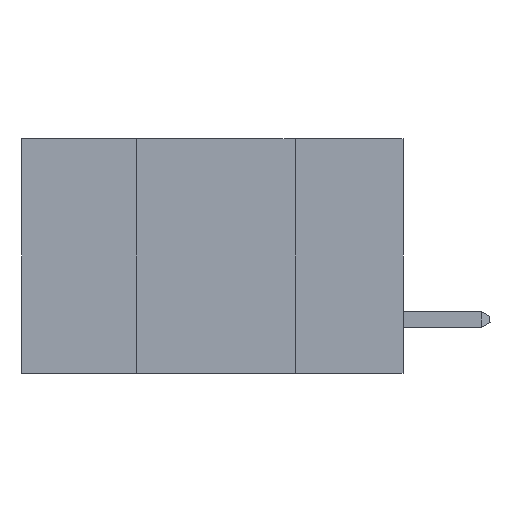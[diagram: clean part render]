
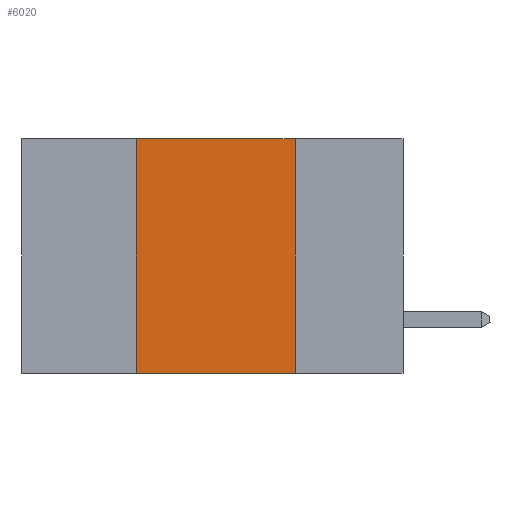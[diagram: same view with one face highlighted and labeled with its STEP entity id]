
A CAD part, left-side view. The second image highlights one B-rep face of the part: STEP entity #6020.
In plain terms, the highlighted planar face has unit normal (-1, 0, 0).
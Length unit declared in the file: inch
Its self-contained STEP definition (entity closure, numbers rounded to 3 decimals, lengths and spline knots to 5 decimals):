
#1434 = LINE ( 'NONE', #20074, #16120 ) ;
#2878 = EDGE_CURVE ( 'NONE', #14919, #8696, #19098, .T. ) ;
#3071 = CARTESIAN_POINT ( 'NONE',  ( 0., 0.17, -0.37 ) ) ;
#3367 = ORIENTED_EDGE ( 'NONE', *, *, #17749, .F. ) ;
#3917 = EDGE_CURVE ( 'NONE', #10066, #10147, #1434, .T. ) ;
#6020 = ADVANCED_FACE ( 'NONE', ( #16825 ), #6338, .F. ) ;
#6338 = PLANE ( 'NONE',  #6796 ) ;
#6494 = DIRECTION ( 'NONE',  ( 0., 0., -1. ) ) ;
#6796 = AXIS2_PLACEMENT_3D ( 'NONE', #10010, #15226, #8141 ) ;
#7015 = CARTESIAN_POINT ( 'NONE',  ( 0., 0.42, 0. ) ) ;
#7322 = EDGE_CURVE ( 'NONE', #14919, #10147, #16235, .T. ) ;
#8141 = DIRECTION ( 'NONE',  ( 0., 0., -1. ) ) ;
#8282 = ORIENTED_EDGE ( 'NONE', *, *, #2878, .F. ) ;
#8696 = VERTEX_POINT ( 'NONE', #7015 ) ;
#8901 = VECTOR ( 'NONE', #17757, 39.37008 ) ;
#10010 = CARTESIAN_POINT ( 'NONE',  ( 0., 0.6, 0. ) ) ;
#10066 = VERTEX_POINT ( 'NONE', #18082 ) ;
#10147 = VERTEX_POINT ( 'NONE', #3071 ) ;
#12273 = CARTESIAN_POINT ( 'NONE',  ( 0., 0.42, 0. ) ) ;
#13842 = ORIENTED_EDGE ( 'NONE', *, *, #7322, .T. ) ;
#14129 = CARTESIAN_POINT ( 'NONE',  ( 0., 0.6, -0.37 ) ) ;
#14497 = CARTESIAN_POINT ( 'NONE',  ( 0., 0.6, 0. ) ) ;
#14919 = VERTEX_POINT ( 'NONE', #20669 ) ;
#15226 = DIRECTION ( 'NONE',  ( 1., 0., 0. ) ) ;
#15530 = EDGE_LOOP ( 'NONE', ( #15555, #3367, #8282, #13842 ) ) ;
#15555 = ORIENTED_EDGE ( 'NONE', *, *, #3917, .F. ) ;
#16120 = VECTOR ( 'NONE', #6494, 39.37008 ) ;
#16235 = LINE ( 'NONE', #14129, #8901 ) ;
#16480 = DIRECTION ( 'NONE',  ( 0., -1., 0. ) ) ;
#16825 = FACE_OUTER_BOUND ( 'NONE', #15530, .T. ) ;
#17749 = EDGE_CURVE ( 'NONE', #8696, #10066, #21459, .T. ) ;
#17757 = DIRECTION ( 'NONE',  ( 0., -1., 0. ) ) ;
#18006 = VECTOR ( 'NONE', #16480, 39.37008 ) ;
#18082 = CARTESIAN_POINT ( 'NONE',  ( 0., 0.17, 0. ) ) ;
#19098 = LINE ( 'NONE', #12273, #21491 ) ;
#19318 = DIRECTION ( 'NONE',  ( 0., 0., 1. ) ) ;
#20074 = CARTESIAN_POINT ( 'NONE',  ( 0., 0.17, 0. ) ) ;
#20669 = CARTESIAN_POINT ( 'NONE',  ( 0., 0.42, -0.37 ) ) ;
#21459 = LINE ( 'NONE', #14497, #18006 ) ;
#21491 = VECTOR ( 'NONE', #19318, 39.37008 ) ;
